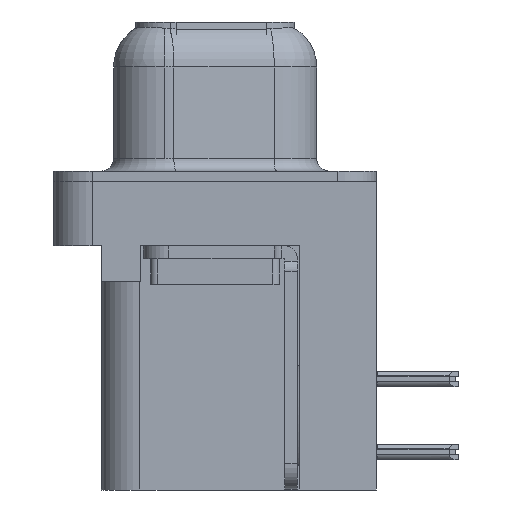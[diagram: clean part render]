
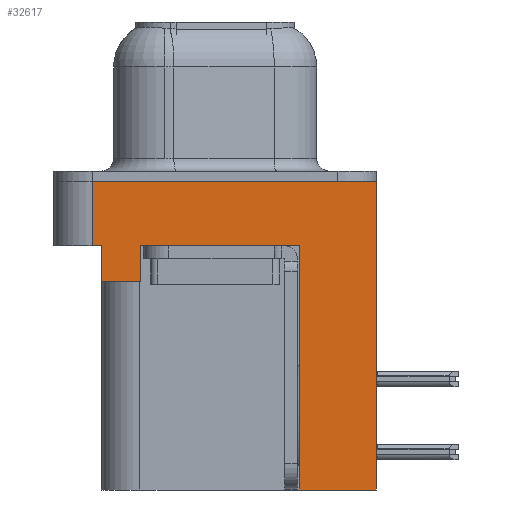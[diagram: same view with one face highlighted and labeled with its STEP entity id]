
A CAD part, left-side view. The second image highlights one B-rep face of the part: STEP entity #32617.
In plain terms, the highlighted planar face has unit normal (-1, 0, 0).
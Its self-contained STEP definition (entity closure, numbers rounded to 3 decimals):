
#258 = VERTEX_POINT ( 'NONE', #20153 ) ;
#574 = DIRECTION ( 'NONE',  ( 0., -1., 0. ) ) ;
#627 = ORIENTED_EDGE ( 'NONE', *, *, #18843, .T. ) ;
#764 = PLANE ( 'NONE',  #1717 ) ;
#840 = CARTESIAN_POINT ( 'NONE',  ( -2.91, -3.295, -12. ) ) ;
#1279 = CARTESIAN_POINT ( 'NONE',  ( -2.91, -6.275, -2.5 ) ) ;
#1717 = AXIS2_PLACEMENT_3D ( 'NONE', #12212, #31349, #3630 ) ;
#1731 = CARTESIAN_POINT ( 'NONE',  ( -2.91, 2.895, -3.9 ) ) ;
#1980 = EDGE_LOOP ( 'NONE', ( #31153, #2332, #31685, #33370, #31905, #22172, #35253, #34793, #14116, #627 ) ) ;
#2241 = CARTESIAN_POINT ( 'NONE',  ( -2.91, 4.425, -3.9 ) ) ;
#2332 = ORIENTED_EDGE ( 'NONE', *, *, #6263, .F. ) ;
#2441 = VECTOR ( 'NONE', #11009, 1000. ) ;
#2485 = VERTEX_POINT ( 'NONE', #7322 ) ;
#3326 = LINE ( 'NONE', #28418, #22059 ) ;
#3630 = DIRECTION ( 'NONE',  ( 0., 0., 1. ) ) ;
#3709 = DIRECTION ( 'NONE',  ( 0., 0., 1. ) ) ;
#3801 = DIRECTION ( 'NONE',  ( 0., -1., 0. ) ) ;
#3806 = LINE ( 'NONE', #8229, #2441 ) ;
#3947 = DIRECTION ( 'NONE',  ( 0., 1., 0. ) ) ;
#4037 = EDGE_CURVE ( 'NONE', #9042, #2485, #33487, .T. ) ;
#4814 = DIRECTION ( 'NONE',  ( 0., 0., 1. ) ) ;
#5043 = CARTESIAN_POINT ( 'NONE',  ( -2.91, 4.775, -2.5 ) ) ;
#6263 = EDGE_CURVE ( 'NONE', #13192, #258, #26271, .T. ) ;
#6641 = VERTEX_POINT ( 'NONE', #32639 ) ;
#7028 = VECTOR ( 'NONE', #18137, 1000. ) ;
#7322 = CARTESIAN_POINT ( 'NONE',  ( -2.91, 2.895, -2.5 ) ) ;
#7356 = CARTESIAN_POINT ( 'NONE',  ( -2.91, 4.425, -3.9 ) ) ;
#7702 = DIRECTION ( 'NONE',  ( 0., 0., 1. ) ) ;
#8204 = VECTOR ( 'NONE', #574, 1000. ) ;
#8229 = CARTESIAN_POINT ( 'NONE',  ( -2.91, -3.295, -12. ) ) ;
#9042 = VERTEX_POINT ( 'NONE', #1731 ) ;
#9426 = LINE ( 'NONE', #17685, #18122 ) ;
#9519 = VERTEX_POINT ( 'NONE', #33386 ) ;
#10171 = VECTOR ( 'NONE', #12924, 1000. ) ;
#10464 = EDGE_CURVE ( 'NONE', #9042, #13300, #27771, .T. ) ;
#11009 = DIRECTION ( 'NONE',  ( 0., 1., 0. ) ) ;
#11536 = VECTOR ( 'NONE', #4814, 1000. ) ;
#11765 = EDGE_CURVE ( 'NONE', #258, #9519, #9426, .T. ) ;
#12212 = CARTESIAN_POINT ( 'NONE',  ( -2.91, -6.275, -2.5 ) ) ;
#12303 = CARTESIAN_POINT ( 'NONE',  ( -2.91, -3.295, -12. ) ) ;
#12924 = DIRECTION ( 'NONE',  ( 0., 0., 1. ) ) ;
#13192 = VERTEX_POINT ( 'NONE', #5043 ) ;
#13300 = VERTEX_POINT ( 'NONE', #2241 ) ;
#14116 = ORIENTED_EDGE ( 'NONE', *, *, #29652, .F. ) ;
#14892 = FACE_OUTER_BOUND ( 'NONE', #1980, .T. ) ;
#15057 = DIRECTION ( 'NONE',  ( 0., -1., 0. ) ) ;
#15198 = VECTOR ( 'NONE', #7702, 1000. ) ;
#15215 = LINE ( 'NONE', #28575, #8204 ) ;
#15850 = EDGE_CURVE ( 'NONE', #13300, #6641, #24658, .T. ) ;
#16066 = VERTEX_POINT ( 'NONE', #22104 ) ;
#16078 = CARTESIAN_POINT ( 'NONE',  ( -2.91, 4.775, -2.5 ) ) ;
#16183 = LINE ( 'NONE', #840, #20906 ) ;
#16593 = CARTESIAN_POINT ( 'NONE',  ( -2.91, -3.295, -2.5 ) ) ;
#17685 = CARTESIAN_POINT ( 'NONE',  ( -2.91, -6.275, 0. ) ) ;
#18122 = VECTOR ( 'NONE', #3801, 1000. ) ;
#18137 = DIRECTION ( 'NONE',  ( 0., 0., 1. ) ) ;
#18843 = EDGE_CURVE ( 'NONE', #16066, #9519, #25689, .T. ) ;
#20153 = CARTESIAN_POINT ( 'NONE',  ( -2.91, 4.775, 0. ) ) ;
#20440 = VECTOR ( 'NONE', #3947, 1000. ) ;
#20906 = VECTOR ( 'NONE', #3709, 1000. ) ;
#22059 = VECTOR ( 'NONE', #15057, 1000. ) ;
#22104 = CARTESIAN_POINT ( 'NONE',  ( -2.91, -6.275, -12. ) ) ;
#22172 = ORIENTED_EDGE ( 'NONE', *, *, #4037, .T. ) ;
#22510 = EDGE_CURVE ( 'NONE', #2485, #34527, #3326, .T. ) ;
#24658 = LINE ( 'NONE', #7356, #15198 ) ;
#25689 = LINE ( 'NONE', #1279, #7028 ) ;
#26271 = LINE ( 'NONE', #16078, #11536 ) ;
#27771 = LINE ( 'NONE', #34193, #20440 ) ;
#28418 = CARTESIAN_POINT ( 'NONE',  ( -2.91, -6.275, -2.5 ) ) ;
#28575 = CARTESIAN_POINT ( 'NONE',  ( -2.91, -6.275, -2.5 ) ) ;
#29202 = CARTESIAN_POINT ( 'NONE',  ( -2.91, 2.895, -3.9 ) ) ;
#29652 = EDGE_CURVE ( 'NONE', #16066, #31608, #3806, .T. ) ;
#31153 = ORIENTED_EDGE ( 'NONE', *, *, #11765, .F. ) ;
#31349 = DIRECTION ( 'NONE',  ( -1., 0., 0. ) ) ;
#31608 = VERTEX_POINT ( 'NONE', #12303 ) ;
#31685 = ORIENTED_EDGE ( 'NONE', *, *, #34847, .T. ) ;
#31905 = ORIENTED_EDGE ( 'NONE', *, *, #10464, .F. ) ;
#32617 = ADVANCED_FACE ( 'NONE', ( #14892 ), #764, .T. ) ;
#32639 = CARTESIAN_POINT ( 'NONE',  ( -2.91, 4.425, -2.5 ) ) ;
#32954 = EDGE_CURVE ( 'NONE', #31608, #34527, #16183, .T. ) ;
#33370 = ORIENTED_EDGE ( 'NONE', *, *, #15850, .F. ) ;
#33386 = CARTESIAN_POINT ( 'NONE',  ( -2.91, -6.275, 0. ) ) ;
#33487 = LINE ( 'NONE', #29202, #10171 ) ;
#34193 = CARTESIAN_POINT ( 'NONE',  ( -2.91, 4.425, -3.9 ) ) ;
#34527 = VERTEX_POINT ( 'NONE', #16593 ) ;
#34793 = ORIENTED_EDGE ( 'NONE', *, *, #32954, .F. ) ;
#34847 = EDGE_CURVE ( 'NONE', #13192, #6641, #15215, .T. ) ;
#35253 = ORIENTED_EDGE ( 'NONE', *, *, #22510, .T. ) ;
